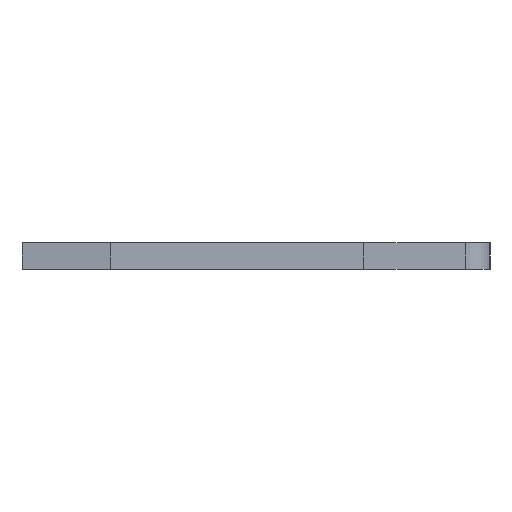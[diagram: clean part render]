
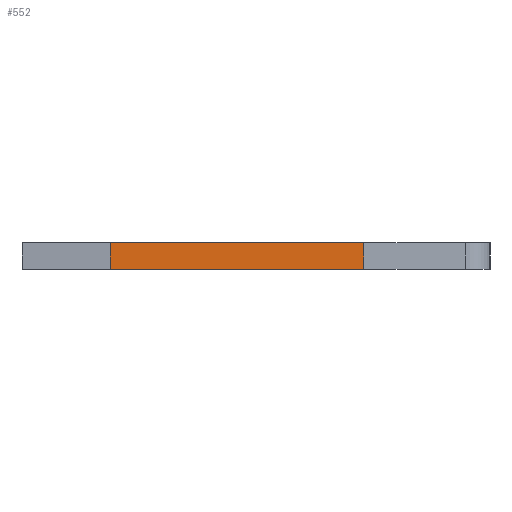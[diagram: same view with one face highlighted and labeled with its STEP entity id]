
A CAD part, left-side view. The second image highlights one B-rep face of the part: STEP entity #552.
In plain terms, the highlighted face is planar.
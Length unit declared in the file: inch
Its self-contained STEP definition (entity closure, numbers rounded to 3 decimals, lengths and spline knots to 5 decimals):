
#28 = LINE ( 'NONE', #519, #121 ) ;
#46 = LINE ( 'NONE', #182, #772 ) ;
#55 = DIRECTION ( 'NONE',  ( 1., 0., 0. ) ) ;
#121 = VECTOR ( 'NONE', #1061, 39.37008 ) ;
#159 = CARTESIAN_POINT ( 'NONE',  ( -0.013, -0.099, -0.0575 ) ) ;
#179 = DIRECTION ( 'NONE',  ( 0., 0., 1. ) ) ;
#182 = CARTESIAN_POINT ( 'NONE',  ( 0.013, 0.146, -0.0575 ) ) ;
#280 = VERTEX_POINT ( 'NONE', #159 ) ;
#299 = CARTESIAN_POINT ( 'NONE',  ( -0.013, 0.146, -0.0575 ) ) ;
#304 = CARTESIAN_POINT ( 'NONE',  ( 0.013, 0.146, -0.0575 ) ) ;
#309 = EDGE_CURVE ( 'NONE', #1670, #472, #702, .T. ) ;
#422 = CARTESIAN_POINT ( 'NONE',  ( 0.013, -0.099, -0.0575 ) ) ;
#468 = CARTESIAN_POINT ( 'NONE',  ( 0.013, -0.099, -0.0575 ) ) ;
#472 = VERTEX_POINT ( 'NONE', #1144 ) ;
#519 = CARTESIAN_POINT ( 'NONE',  ( -0.013, 0.146, -0.0575 ) ) ;
#552 = ADVANCED_FACE ( 'NONE', ( #733 ), #1044, .F. ) ;
#685 = ORIENTED_EDGE ( 'NONE', *, *, #899, .T. ) ;
#702 = LINE ( 'NONE', #304, #919 ) ;
#703 = EDGE_CURVE ( 'NONE', #472, #1779, #46, .T. ) ;
#733 = FACE_OUTER_BOUND ( 'NONE', #939, .T. ) ;
#772 = VECTOR ( 'NONE', #1171, 39.37008 ) ;
#899 = EDGE_CURVE ( 'NONE', #280, #1779, #28, .T. ) ;
#916 = CARTESIAN_POINT ( 'NONE',  ( 0.013, 0.146, -0.0575 ) ) ;
#919 = VECTOR ( 'NONE', #1016, 39.37008 ) ;
#939 = EDGE_LOOP ( 'NONE', ( #685, #957, #1438, #1284 ) ) ;
#957 = ORIENTED_EDGE ( 'NONE', *, *, #703, .F. ) ;
#1016 = DIRECTION ( 'NONE',  ( 0., 1., 0. ) ) ;
#1044 = PLANE ( 'NONE',  #1537 ) ;
#1061 = DIRECTION ( 'NONE',  ( 0., 1., 0. ) ) ;
#1144 = CARTESIAN_POINT ( 'NONE',  ( 0.013, 0.146, -0.0575 ) ) ;
#1171 = DIRECTION ( 'NONE',  ( -1., 0., 0. ) ) ;
#1284 = ORIENTED_EDGE ( 'NONE', *, *, #1633, .T. ) ;
#1438 = ORIENTED_EDGE ( 'NONE', *, *, #309, .F. ) ;
#1447 = VECTOR ( 'NONE', #1551, 39.37008 ) ;
#1537 = AXIS2_PLACEMENT_3D ( 'NONE', #916, #179, #55 ) ;
#1551 = DIRECTION ( 'NONE',  ( -1., 0., 0. ) ) ;
#1574 = LINE ( 'NONE', #422, #1447 ) ;
#1633 = EDGE_CURVE ( 'NONE', #1670, #280, #1574, .T. ) ;
#1670 = VERTEX_POINT ( 'NONE', #468 ) ;
#1779 = VERTEX_POINT ( 'NONE', #299 ) ;
